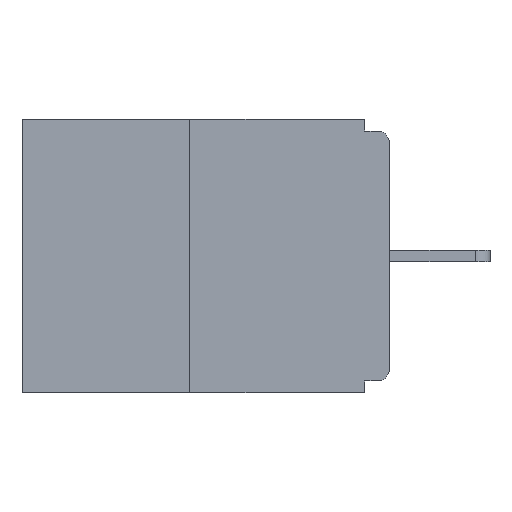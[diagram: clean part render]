
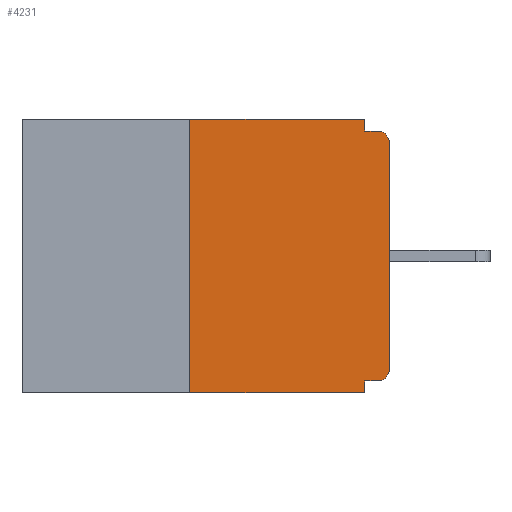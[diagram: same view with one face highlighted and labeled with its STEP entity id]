
A CAD part, left-side view. The second image highlights one B-rep face of the part: STEP entity #4231.
In plain terms, the highlighted planar face has unit normal (-1, 0, 0).
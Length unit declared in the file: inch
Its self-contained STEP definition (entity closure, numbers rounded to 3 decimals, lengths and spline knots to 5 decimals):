
#275 = VECTOR ( 'NONE', #7231, 39.37008 ) ;
#281 = CARTESIAN_POINT ( 'NONE',  ( 0., 0.015, -0.03 ) ) ;
#327 = LINE ( 'NONE', #9381, #6682 ) ;
#343 = DIRECTION ( 'NONE',  ( 1., 0., 0. ) ) ;
#360 = EDGE_CURVE ( 'NONE', #9391, #7001, #4966, .T. ) ;
#430 = EDGE_CURVE ( 'NONE', #9391, #7041, #5396, .T. ) ;
#501 = ORIENTED_EDGE ( 'NONE', *, *, #683, .T. ) ;
#683 = EDGE_CURVE ( 'NONE', #7041, #6365, #327, .T. ) ;
#779 = VECTOR ( 'NONE', #2112, 39.37008 ) ;
#918 = LINE ( 'NONE', #10026, #6854 ) ;
#936 = LINE ( 'NONE', #3357, #10153 ) ;
#954 = DIRECTION ( 'NONE',  ( 0., 0., -1. ) ) ;
#1023 = VECTOR ( 'NONE', #5523, 39.37008 ) ;
#1108 = ORIENTED_EDGE ( 'NONE', *, *, #3537, .T. ) ;
#1110 = DIRECTION ( 'NONE',  ( 0., 0., -1. ) ) ;
#1278 = LINE ( 'NONE', #10326, #275 ) ;
#1645 = ORIENTED_EDGE ( 'NONE', *, *, #9345, .F. ) ;
#1917 = DIRECTION ( 'NONE',  ( -1., 0., 0. ) ) ;
#2020 = VERTEX_POINT ( 'NONE', #7600 ) ;
#2112 = DIRECTION ( 'NONE',  ( 0., -1., 0. ) ) ;
#2700 = ORIENTED_EDGE ( 'NONE', *, *, #360, .F. ) ;
#2969 = FACE_OUTER_BOUND ( 'NONE', #10216, .T. ) ;
#2989 = CARTESIAN_POINT ( 'NONE',  ( 0., 0.031, -0.328 ) ) ;
#3212 = CARTESIAN_POINT ( 'NONE',  ( 0., 0., -0.328 ) ) ;
#3357 = CARTESIAN_POINT ( 'NONE',  ( 0., 0.031, -0.343 ) ) ;
#3537 = EDGE_CURVE ( 'NONE', #6365, #6597, #3933, .T. ) ;
#3636 = CARTESIAN_POINT ( 'NONE',  ( 0., 0.015, -0.313 ) ) ;
#3793 = DIRECTION ( 'NONE',  ( 0., 0., -1. ) ) ;
#3865 = ORIENTED_EDGE ( 'NONE', *, *, #430, .T. ) ;
#3933 = CIRCLE ( 'NONE', #4304, 0.015 ) ;
#4154 = EDGE_CURVE ( 'NONE', #7001, #4211, #936, .T. ) ;
#4200 = ORIENTED_EDGE ( 'NONE', *, *, #6643, .F. ) ;
#4211 = VERTEX_POINT ( 'NONE', #10190 ) ;
#4223 = ORIENTED_EDGE ( 'NONE', *, *, #8346, .T. ) ;
#4231 = ADVANCED_FACE ( 'NONE', ( #2969 ), #7039, .F. ) ;
#4251 = DIRECTION ( 'NONE',  ( 0., 0., -1. ) ) ;
#4261 = DIRECTION ( 'NONE',  ( 0., 1., 0. ) ) ;
#4304 = AXIS2_PLACEMENT_3D ( 'NONE', #281, #5329, #5385 ) ;
#4966 = LINE ( 'NONE', #3212, #8289 ) ;
#5329 = DIRECTION ( 'NONE',  ( -1., 0., 0. ) ) ;
#5385 = DIRECTION ( 'NONE',  ( 0., 0., -1. ) ) ;
#5396 = CIRCLE ( 'NONE', #6758, 0.015 ) ;
#5523 = DIRECTION ( 'NONE',  ( 0., -1., 0. ) ) ;
#6043 = LINE ( 'NONE', #10248, #779 ) ;
#6307 = LINE ( 'NONE', #9563, #1023 ) ;
#6365 = VERTEX_POINT ( 'NONE', #8733 ) ;
#6387 = CARTESIAN_POINT ( 'NONE',  ( 0., 0.015, -0.015 ) ) ;
#6557 = CARTESIAN_POINT ( 'NONE',  ( 0., 0.25, 0. ) ) ;
#6578 = CARTESIAN_POINT ( 'NONE',  ( 0., 0., -0.313 ) ) ;
#6597 = VERTEX_POINT ( 'NONE', #6387 ) ;
#6643 = EDGE_CURVE ( 'NONE', #7954, #2020, #8454, .T. ) ;
#6658 = DIRECTION ( 'NONE',  ( 0., -1., 0. ) ) ;
#6682 = VECTOR ( 'NONE', #6767, 39.37008 ) ;
#6758 = AXIS2_PLACEMENT_3D ( 'NONE', #3636, #1917, #1110 ) ;
#6767 = DIRECTION ( 'NONE',  ( 0., 0., 1. ) ) ;
#6816 = ORIENTED_EDGE ( 'NONE', *, *, #10223, .F. ) ;
#6854 = VECTOR ( 'NONE', #6658, 39.37008 ) ;
#7001 = VERTEX_POINT ( 'NONE', #2989 ) ;
#7019 = EDGE_CURVE ( 'NONE', #2020, #6597, #6307, .T. ) ;
#7039 = PLANE ( 'NONE',  #7585 ) ;
#7041 = VERTEX_POINT ( 'NONE', #6578 ) ;
#7149 = CARTESIAN_POINT ( 'NONE',  ( 0., 0.25, -0.343 ) ) ;
#7184 = ORIENTED_EDGE ( 'NONE', *, *, #7019, .F. ) ;
#7231 = DIRECTION ( 'NONE',  ( 0., 0., 1. ) ) ;
#7287 = VECTOR ( 'NONE', #954, 39.37008 ) ;
#7585 = AXIS2_PLACEMENT_3D ( 'NONE', #8762, #343, #3793 ) ;
#7600 = CARTESIAN_POINT ( 'NONE',  ( 0., 0.031, -0.015 ) ) ;
#7648 = CARTESIAN_POINT ( 'NONE',  ( 0., 0.031, 0. ) ) ;
#7852 = CARTESIAN_POINT ( 'NONE',  ( 0., 0.031, 0. ) ) ;
#7954 = VERTEX_POINT ( 'NONE', #7852 ) ;
#8289 = VECTOR ( 'NONE', #4261, 39.37008 ) ;
#8346 = EDGE_CURVE ( 'NONE', #8506, #4211, #6043, .T. ) ;
#8454 = LINE ( 'NONE', #7648, #7287 ) ;
#8506 = VERTEX_POINT ( 'NONE', #7149 ) ;
#8733 = CARTESIAN_POINT ( 'NONE',  ( 0., 0., -0.03 ) ) ;
#8762 = CARTESIAN_POINT ( 'NONE',  ( 0., 0.46, 0. ) ) ;
#8785 = ORIENTED_EDGE ( 'NONE', *, *, #4154, .F. ) ;
#9345 = EDGE_CURVE ( 'NONE', #8506, #10237, #1278, .T. ) ;
#9381 = CARTESIAN_POINT ( 'NONE',  ( 0., 0., 0. ) ) ;
#9391 = VERTEX_POINT ( 'NONE', #9636 ) ;
#9563 = CARTESIAN_POINT ( 'NONE',  ( 0., 0., -0.015 ) ) ;
#9636 = CARTESIAN_POINT ( 'NONE',  ( 0., 0.015, -0.328 ) ) ;
#10026 = CARTESIAN_POINT ( 'NONE',  ( 0., 0.46, 0. ) ) ;
#10153 = VECTOR ( 'NONE', #4251, 39.37008 ) ;
#10190 = CARTESIAN_POINT ( 'NONE',  ( 0., 0.031, -0.343 ) ) ;
#10216 = EDGE_LOOP ( 'NONE', ( #6816, #1645, #4223, #8785, #2700, #3865, #501, #1108, #7184, #4200 ) ) ;
#10223 = EDGE_CURVE ( 'NONE', #10237, #7954, #918, .T. ) ;
#10237 = VERTEX_POINT ( 'NONE', #6557 ) ;
#10248 = CARTESIAN_POINT ( 'NONE',  ( 0., 0.46, -0.343 ) ) ;
#10326 = CARTESIAN_POINT ( 'NONE',  ( 0., 0.25, 0. ) ) ;
